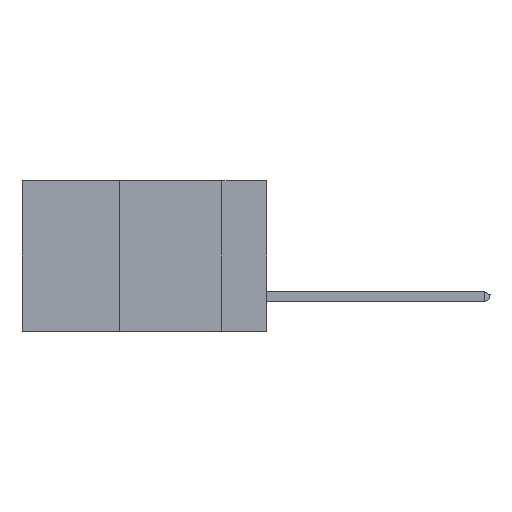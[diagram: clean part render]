
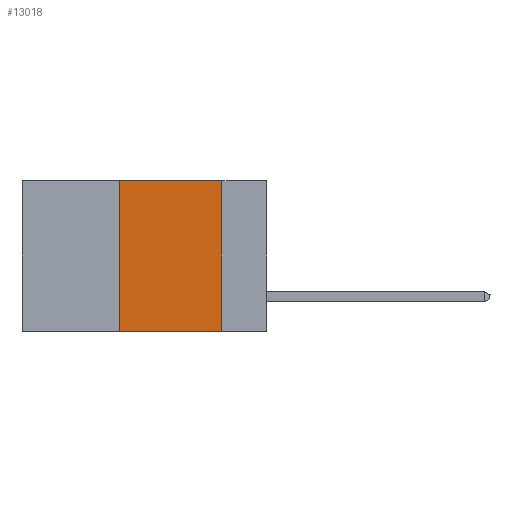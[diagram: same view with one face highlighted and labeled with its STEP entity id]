
A CAD part, left-side view. The second image highlights one B-rep face of the part: STEP entity #13018.
In plain terms, the highlighted planar face has unit normal (-1, 0, 0).
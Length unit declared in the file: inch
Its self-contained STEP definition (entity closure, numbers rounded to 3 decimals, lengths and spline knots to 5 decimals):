
#599 = ORIENTED_EDGE ( 'NONE', *, *, #10135, .F. ) ;
#2345 = EDGE_CURVE ( 'NONE', #4003, #16175, #9676, .T. ) ;
#2645 = CARTESIAN_POINT ( 'NONE',  ( 0., 0.6, 0. ) ) ;
#2961 = EDGE_LOOP ( 'NONE', ( #9107, #20488, #599, #11891 ) ) ;
#2996 = CARTESIAN_POINT ( 'NONE',  ( 0., 0.11, -0.37 ) ) ;
#3307 = DIRECTION ( 'NONE',  ( 0., -1., 0. ) ) ;
#3410 = LINE ( 'NONE', #24745, #22405 ) ;
#3473 = EDGE_CURVE ( 'NONE', #16574, #10582, #18733, .T. ) ;
#4003 = VERTEX_POINT ( 'NONE', #12075 ) ;
#4673 = LINE ( 'NONE', #8499, #18356 ) ;
#5131 = EDGE_CURVE ( 'NONE', #10582, #16175, #3410, .T. ) ;
#6127 = AXIS2_PLACEMENT_3D ( 'NONE', #2645, #12146, #12030 ) ;
#7022 = CARTESIAN_POINT ( 'NONE',  ( 0., 0.6, 0. ) ) ;
#7946 = VECTOR ( 'NONE', #3307, 39.37008 ) ;
#8499 = CARTESIAN_POINT ( 'NONE',  ( 0., 0.36, 0. ) ) ;
#9107 = ORIENTED_EDGE ( 'NONE', *, *, #5131, .F. ) ;
#9676 = LINE ( 'NONE', #19237, #24635 ) ;
#10135 = EDGE_CURVE ( 'NONE', #4003, #16574, #4673, .T. ) ;
#10582 = VERTEX_POINT ( 'NONE', #23541 ) ;
#11142 = CARTESIAN_POINT ( 'NONE',  ( 0., 0.36, 0. ) ) ;
#11891 = ORIENTED_EDGE ( 'NONE', *, *, #2345, .T. ) ;
#12030 = DIRECTION ( 'NONE',  ( 0., 0., -1. ) ) ;
#12075 = CARTESIAN_POINT ( 'NONE',  ( 0., 0.36, -0.37 ) ) ;
#12146 = DIRECTION ( 'NONE',  ( 1., 0., 0. ) ) ;
#13018 = ADVANCED_FACE ( 'NONE', ( #13822 ), #17819, .F. ) ;
#13822 = FACE_OUTER_BOUND ( 'NONE', #2961, .T. ) ;
#16107 = DIRECTION ( 'NONE',  ( 0., 0., 1. ) ) ;
#16175 = VERTEX_POINT ( 'NONE', #2996 ) ;
#16574 = VERTEX_POINT ( 'NONE', #11142 ) ;
#16639 = DIRECTION ( 'NONE',  ( 0., 0., -1. ) ) ;
#17819 = PLANE ( 'NONE',  #6127 ) ;
#18356 = VECTOR ( 'NONE', #16107, 39.37008 ) ;
#18733 = LINE ( 'NONE', #7022, #7946 ) ;
#19237 = CARTESIAN_POINT ( 'NONE',  ( 0., 0.6, -0.37 ) ) ;
#20488 = ORIENTED_EDGE ( 'NONE', *, *, #3473, .F. ) ;
#22405 = VECTOR ( 'NONE', #16639, 39.37008 ) ;
#23084 = DIRECTION ( 'NONE',  ( 0., -1., 0. ) ) ;
#23541 = CARTESIAN_POINT ( 'NONE',  ( 0., 0.11, 0. ) ) ;
#24635 = VECTOR ( 'NONE', #23084, 39.37008 ) ;
#24745 = CARTESIAN_POINT ( 'NONE',  ( 0., 0.11, 0. ) ) ;
